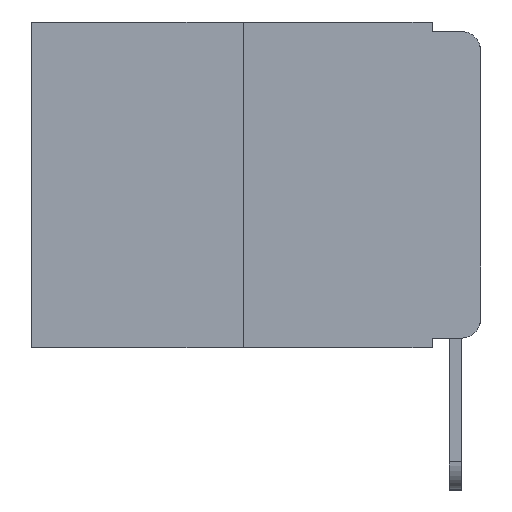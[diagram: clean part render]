
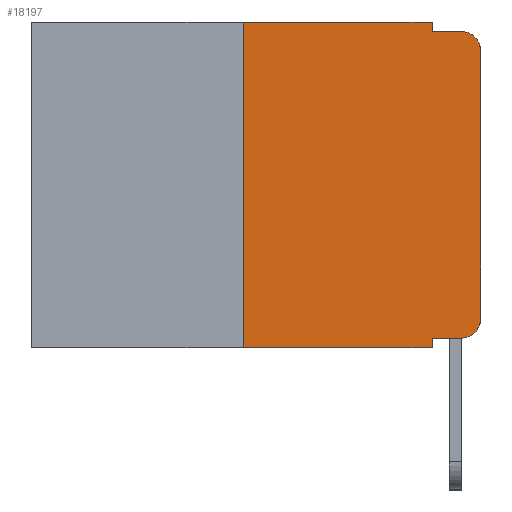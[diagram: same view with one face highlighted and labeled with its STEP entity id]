
A CAD part, left-side view. The second image highlights one B-rep face of the part: STEP entity #18197.
In plain terms, the highlighted planar face has unit normal (-1, 0, 0).
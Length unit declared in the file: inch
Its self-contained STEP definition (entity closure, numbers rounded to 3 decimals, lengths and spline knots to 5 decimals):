
#345 = DIRECTION ( 'NONE',  ( 0., 0., 1. ) ) ;
#551 = AXIS2_PLACEMENT_3D ( 'NONE', #11674, #2227, #7698 ) ;
#730 = EDGE_CURVE ( 'NONE', #4716, #15964, #24777, .T. ) ;
#752 = CARTESIAN_POINT ( 'NONE',  ( 0., 0.25, 0. ) ) ;
#946 = ORIENTED_EDGE ( 'NONE', *, *, #12564, .T. ) ;
#1165 = VECTOR ( 'NONE', #23712, 39.37008 ) ;
#1423 = LINE ( 'NONE', #24534, #21302 ) ;
#2227 = DIRECTION ( 'NONE',  ( -1., 0., 0. ) ) ;
#4037 = DIRECTION ( 'NONE',  ( 0., -1., 0. ) ) ;
#4127 = VECTOR ( 'NONE', #8502, 39.37008 ) ;
#4254 = CARTESIAN_POINT ( 'NONE',  ( 0., 0., -0.03 ) ) ;
#4346 = EDGE_CURVE ( 'NONE', #19708, #9740, #13689, .T. ) ;
#4716 = VERTEX_POINT ( 'NONE', #19832 ) ;
#4794 = LINE ( 'NONE', #12301, #1165 ) ;
#4859 = CARTESIAN_POINT ( 'NONE',  ( 0., 0.473, 0. ) ) ;
#5488 = VERTEX_POINT ( 'NONE', #23134 ) ;
#5532 = DIRECTION ( 'NONE',  ( 0., -1., 0. ) ) ;
#5712 = CARTESIAN_POINT ( 'NONE',  ( 0., 0.051, -0.01 ) ) ;
#6425 = ORIENTED_EDGE ( 'NONE', *, *, #6537, .T. ) ;
#6537 = EDGE_CURVE ( 'NONE', #8463, #5488, #12076, .T. ) ;
#6731 = DIRECTION ( 'NONE',  ( 0., 0., -1. ) ) ;
#6909 = LINE ( 'NONE', #4859, #14698 ) ;
#7236 = VECTOR ( 'NONE', #14518, 39.37008 ) ;
#7698 = DIRECTION ( 'NONE',  ( 0., 0., -1. ) ) ;
#8463 = VERTEX_POINT ( 'NONE', #21049 ) ;
#8502 = DIRECTION ( 'NONE',  ( 0., 0., 1. ) ) ;
#8722 = LINE ( 'NONE', #23999, #7236 ) ;
#8956 = FACE_OUTER_BOUND ( 'NONE', #11148, .T. ) ;
#9136 = VECTOR ( 'NONE', #18100, 39.37008 ) ;
#9511 = AXIS2_PLACEMENT_3D ( 'NONE', #21045, #23119, #11394 ) ;
#9740 = VERTEX_POINT ( 'NONE', #14256 ) ;
#10269 = CARTESIAN_POINT ( 'NONE',  ( 0., 0.02, -0.03 ) ) ;
#10339 = ORIENTED_EDGE ( 'NONE', *, *, #20976, .T. ) ;
#10838 = CARTESIAN_POINT ( 'NONE',  ( 0., 0.051, -0.343 ) ) ;
#11148 = EDGE_LOOP ( 'NONE', ( #23109, #946, #12375, #22839, #23611, #14069, #10339, #20254, #20099, #6425 ) ) ;
#11377 = CIRCLE ( 'NONE', #18628, 0.02 ) ;
#11394 = DIRECTION ( 'NONE',  ( 0., 0., -1. ) ) ;
#11674 = CARTESIAN_POINT ( 'NONE',  ( 0., 0.02, -0.313 ) ) ;
#12076 = CIRCLE ( 'NONE', #551, 0.02 ) ;
#12301 = CARTESIAN_POINT ( 'NONE',  ( 0., 0.051, 0. ) ) ;
#12312 = CARTESIAN_POINT ( 'NONE',  ( 0., 0.02, -0.01 ) ) ;
#12375 = ORIENTED_EDGE ( 'NONE', *, *, #18695, .F. ) ;
#12564 = EDGE_CURVE ( 'NONE', #14191, #17731, #11377, .T. ) ;
#13231 = CARTESIAN_POINT ( 'NONE',  ( 0., 0.051, -0.333 ) ) ;
#13561 = PLANE ( 'NONE',  #9511 ) ;
#13689 = LINE ( 'NONE', #752, #4127 ) ;
#13767 = LINE ( 'NONE', #13231, #14670 ) ;
#14069 = ORIENTED_EDGE ( 'NONE', *, *, #4346, .F. ) ;
#14191 = VERTEX_POINT ( 'NONE', #4254 ) ;
#14256 = CARTESIAN_POINT ( 'NONE',  ( 0., 0.25, 0. ) ) ;
#14518 = DIRECTION ( 'NONE',  ( 0., -1., 0. ) ) ;
#14670 = VECTOR ( 'NONE', #4037, 39.37008 ) ;
#14698 = VECTOR ( 'NONE', #18327, 39.37008 ) ;
#15514 = CARTESIAN_POINT ( 'NONE',  ( 0., 0.051, -0.333 ) ) ;
#15964 = VERTEX_POINT ( 'NONE', #5712 ) ;
#17219 = EDGE_CURVE ( 'NONE', #21865, #21036, #4794, .T. ) ;
#17721 = CARTESIAN_POINT ( 'NONE',  ( 0., 0., 0. ) ) ;
#17731 = VERTEX_POINT ( 'NONE', #12312 ) ;
#18100 = DIRECTION ( 'NONE',  ( 0., 0., -1. ) ) ;
#18197 = ADVANCED_FACE ( 'NONE', ( #8956 ), #13561, .F. ) ;
#18327 = DIRECTION ( 'NONE',  ( 0., -1., 0. ) ) ;
#18628 = AXIS2_PLACEMENT_3D ( 'NONE', #10269, #19970, #6731 ) ;
#18695 = EDGE_CURVE ( 'NONE', #15964, #17731, #1423, .T. ) ;
#18854 = LINE ( 'NONE', #17721, #19441 ) ;
#19441 = VECTOR ( 'NONE', #345, 39.37008 ) ;
#19708 = VERTEX_POINT ( 'NONE', #23174 ) ;
#19832 = CARTESIAN_POINT ( 'NONE',  ( 0., 0.051, 0. ) ) ;
#19970 = DIRECTION ( 'NONE',  ( -1., 0., 0. ) ) ;
#20099 = ORIENTED_EDGE ( 'NONE', *, *, #22653, .T. ) ;
#20197 = CARTESIAN_POINT ( 'NONE',  ( 0., 0.051, 0. ) ) ;
#20254 = ORIENTED_EDGE ( 'NONE', *, *, #17219, .F. ) ;
#20976 = EDGE_CURVE ( 'NONE', #19708, #21036, #8722, .T. ) ;
#21036 = VERTEX_POINT ( 'NONE', #10838 ) ;
#21045 = CARTESIAN_POINT ( 'NONE',  ( 0., 0.473, 0. ) ) ;
#21049 = CARTESIAN_POINT ( 'NONE',  ( 0., 0.02, -0.333 ) ) ;
#21302 = VECTOR ( 'NONE', #5532, 39.37008 ) ;
#21865 = VERTEX_POINT ( 'NONE', #15514 ) ;
#22391 = EDGE_CURVE ( 'NONE', #9740, #4716, #6909, .T. ) ;
#22653 = EDGE_CURVE ( 'NONE', #21865, #8463, #13767, .T. ) ;
#22839 = ORIENTED_EDGE ( 'NONE', *, *, #730, .F. ) ;
#23109 = ORIENTED_EDGE ( 'NONE', *, *, #24601, .T. ) ;
#23119 = DIRECTION ( 'NONE',  ( 1., 0., 0. ) ) ;
#23134 = CARTESIAN_POINT ( 'NONE',  ( 0., 0., -0.313 ) ) ;
#23174 = CARTESIAN_POINT ( 'NONE',  ( 0., 0.25, -0.343 ) ) ;
#23611 = ORIENTED_EDGE ( 'NONE', *, *, #22391, .F. ) ;
#23712 = DIRECTION ( 'NONE',  ( 0., 0., -1. ) ) ;
#23999 = CARTESIAN_POINT ( 'NONE',  ( 0., 0.473, -0.343 ) ) ;
#24534 = CARTESIAN_POINT ( 'NONE',  ( 0., 0.051, -0.01 ) ) ;
#24601 = EDGE_CURVE ( 'NONE', #5488, #14191, #18854, .T. ) ;
#24777 = LINE ( 'NONE', #20197, #9136 ) ;
